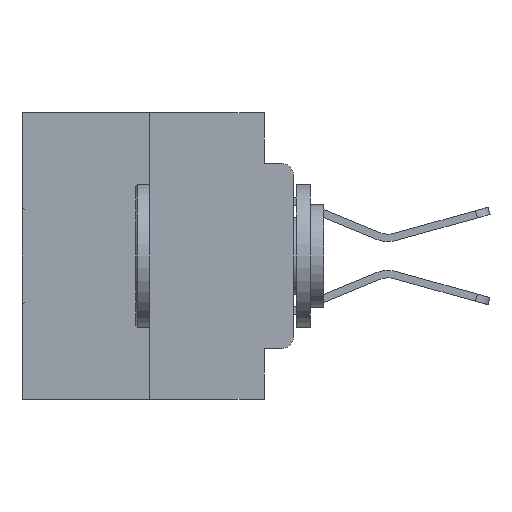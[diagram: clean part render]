
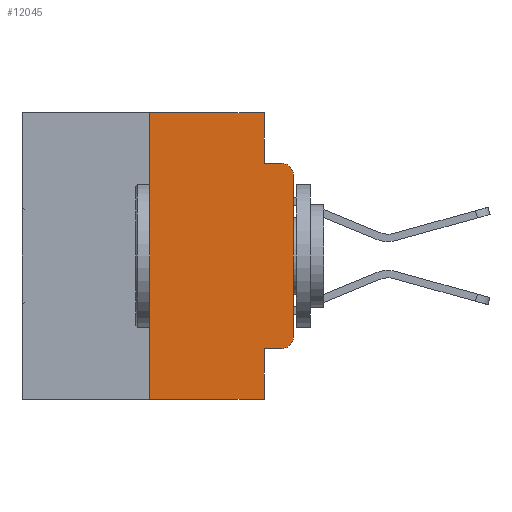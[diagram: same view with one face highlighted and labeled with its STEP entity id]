
A CAD part, left-side view. The second image highlights one B-rep face of the part: STEP entity #12045.
In plain terms, the highlighted planar face has unit normal (-1, 0, 0).
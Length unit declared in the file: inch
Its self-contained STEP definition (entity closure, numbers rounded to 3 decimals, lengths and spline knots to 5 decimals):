
#248 = ORIENTED_EDGE ( 'NONE', *, *, #29939, .F. ) ;
#392 = CARTESIAN_POINT ( 'NONE',  ( 0., 0.25, 0. ) ) ;
#1070 = VERTEX_POINT ( 'NONE', #29935 ) ;
#1841 = VECTOR ( 'NONE', #20340, 39.37008 ) ;
#1913 = CARTESIAN_POINT ( 'NONE',  ( 0., 0.051, -0.0885 ) ) ;
#2351 = CIRCLE ( 'NONE', #13292, 0.02 ) ;
#2921 = CARTESIAN_POINT ( 'NONE',  ( 0., 0.051, -0.4115 ) ) ;
#3362 = CIRCLE ( 'NONE', #20977, 0.02 ) ;
#3447 = ORIENTED_EDGE ( 'NONE', *, *, #20067, .F. ) ;
#3627 = CARTESIAN_POINT ( 'NONE',  ( 0., 0., -0.1085 ) ) ;
#3645 = VECTOR ( 'NONE', #14641, 39.37008 ) ;
#3833 = ORIENTED_EDGE ( 'NONE', *, *, #9875, .T. ) ;
#3964 = CARTESIAN_POINT ( 'NONE',  ( 0., 0.25, 0. ) ) ;
#4243 = ORIENTED_EDGE ( 'NONE', *, *, #16883, .T. ) ;
#4433 = LINE ( 'NONE', #17026, #3645 ) ;
#4945 = DIRECTION ( 'NONE',  ( 0., 0., -1. ) ) ;
#5518 = LINE ( 'NONE', #28507, #30923 ) ;
#5643 = CARTESIAN_POINT ( 'NONE',  ( 0., 0.051, -0.5 ) ) ;
#6597 = VECTOR ( 'NONE', #8872, 39.37008 ) ;
#6677 = VERTEX_POINT ( 'NONE', #2921 ) ;
#7301 = EDGE_CURVE ( 'NONE', #14435, #19936, #5518, .T. ) ;
#7581 = CARTESIAN_POINT ( 'NONE',  ( 0., 0.051, 0. ) ) ;
#8117 = VERTEX_POINT ( 'NONE', #5643 ) ;
#8255 = EDGE_CURVE ( 'NONE', #21216, #1070, #2351, .T. ) ;
#8353 = LINE ( 'NONE', #15565, #1841 ) ;
#8384 = ORIENTED_EDGE ( 'NONE', *, *, #28106, .F. ) ;
#8458 = CARTESIAN_POINT ( 'NONE',  ( 0., 0.051, 0. ) ) ;
#8872 = DIRECTION ( 'NONE',  ( 0., 0., -1. ) ) ;
#9291 = CARTESIAN_POINT ( 'NONE',  ( 0., 0.02, -0.4115 ) ) ;
#9875 = EDGE_CURVE ( 'NONE', #13082, #21216, #8353, .T. ) ;
#10429 = LINE ( 'NONE', #13683, #28762 ) ;
#11881 = DIRECTION ( 'NONE',  ( -1., 0., 0. ) ) ;
#11978 = CARTESIAN_POINT ( 'NONE',  ( 0., 0.473, 0. ) ) ;
#12045 = ADVANCED_FACE ( 'NONE', ( #12882 ), #16904, .F. ) ;
#12492 = DIRECTION ( 'NONE',  ( 0., -1., 0. ) ) ;
#12882 = FACE_OUTER_BOUND ( 'NONE', #13232, .T. ) ;
#13082 = VERTEX_POINT ( 'NONE', #24380 ) ;
#13232 = EDGE_LOOP ( 'NONE', ( #3833, #17347, #248, #13244, #26715, #8384, #21095, #3447, #22597, #4243 ) ) ;
#13244 = ORIENTED_EDGE ( 'NONE', *, *, #29693, .F. ) ;
#13292 = AXIS2_PLACEMENT_3D ( 'NONE', #27724, #13378, #30105 ) ;
#13378 = DIRECTION ( 'NONE',  ( -1., 0., 0. ) ) ;
#13556 = DIRECTION ( 'NONE',  ( 0., 0., 1. ) ) ;
#13683 = CARTESIAN_POINT ( 'NONE',  ( 0., 0.473, -0.5 ) ) ;
#14181 = DIRECTION ( 'NONE',  ( 0., -1., 0. ) ) ;
#14435 = VERTEX_POINT ( 'NONE', #392 ) ;
#14641 = DIRECTION ( 'NONE',  ( 0., -1., 0. ) ) ;
#15565 = CARTESIAN_POINT ( 'NONE',  ( 0., 0., 0. ) ) ;
#16262 = VERTEX_POINT ( 'NONE', #9291 ) ;
#16663 = VERTEX_POINT ( 'NONE', #20560 ) ;
#16883 = EDGE_CURVE ( 'NONE', #16262, #13082, #3362, .T. ) ;
#16904 = PLANE ( 'NONE',  #25812 ) ;
#17026 = CARTESIAN_POINT ( 'NONE',  ( 0., 0.051, -0.4115 ) ) ;
#17347 = ORIENTED_EDGE ( 'NONE', *, *, #8255, .T. ) ;
#18470 = EDGE_CURVE ( 'NONE', #6677, #16262, #4433, .T. ) ;
#19302 = DIRECTION ( 'NONE',  ( 1., 0., 0. ) ) ;
#19936 = VERTEX_POINT ( 'NONE', #8458 ) ;
#20067 = EDGE_CURVE ( 'NONE', #6677, #8117, #26420, .T. ) ;
#20340 = DIRECTION ( 'NONE',  ( 0., 0., 1. ) ) ;
#20560 = CARTESIAN_POINT ( 'NONE',  ( 0., 0.25, -0.5 ) ) ;
#20977 = AXIS2_PLACEMENT_3D ( 'NONE', #26201, #11881, #28626 ) ;
#21095 = ORIENTED_EDGE ( 'NONE', *, *, #25708, .T. ) ;
#21216 = VERTEX_POINT ( 'NONE', #3627 ) ;
#21858 = LINE ( 'NONE', #7581, #27489 ) ;
#22597 = ORIENTED_EDGE ( 'NONE', *, *, #18470, .T. ) ;
#24380 = CARTESIAN_POINT ( 'NONE',  ( 0., 0., -0.3915 ) ) ;
#24541 = LINE ( 'NONE', #3964, #30844 ) ;
#25602 = CARTESIAN_POINT ( 'NONE',  ( 0., 0.051, 0. ) ) ;
#25708 = EDGE_CURVE ( 'NONE', #16663, #8117, #10429, .T. ) ;
#25812 = AXIS2_PLACEMENT_3D ( 'NONE', #11978, #19302, #4945 ) ;
#26201 = CARTESIAN_POINT ( 'NONE',  ( 0., 0.02, -0.3915 ) ) ;
#26246 = VECTOR ( 'NONE', #12492, 39.37008 ) ;
#26420 = LINE ( 'NONE', #25602, #6597 ) ;
#26715 = ORIENTED_EDGE ( 'NONE', *, *, #7301, .F. ) ;
#26999 = LINE ( 'NONE', #29329, #26246 ) ;
#27489 = VECTOR ( 'NONE', #29133, 39.37008 ) ;
#27544 = VERTEX_POINT ( 'NONE', #1913 ) ;
#27724 = CARTESIAN_POINT ( 'NONE',  ( 0., 0.02, -0.1085 ) ) ;
#27998 = DIRECTION ( 'NONE',  ( 0., -1., 0. ) ) ;
#28106 = EDGE_CURVE ( 'NONE', #16663, #14435, #24541, .T. ) ;
#28507 = CARTESIAN_POINT ( 'NONE',  ( 0., 0.473, 0. ) ) ;
#28626 = DIRECTION ( 'NONE',  ( 0., 0., -1. ) ) ;
#28762 = VECTOR ( 'NONE', #27998, 39.37008 ) ;
#29133 = DIRECTION ( 'NONE',  ( 0., 0., -1. ) ) ;
#29329 = CARTESIAN_POINT ( 'NONE',  ( 0., 0.051, -0.0885 ) ) ;
#29693 = EDGE_CURVE ( 'NONE', #19936, #27544, #21858, .T. ) ;
#29935 = CARTESIAN_POINT ( 'NONE',  ( 0., 0.02, -0.0885 ) ) ;
#29939 = EDGE_CURVE ( 'NONE', #27544, #1070, #26999, .T. ) ;
#30105 = DIRECTION ( 'NONE',  ( 0., 0., -1. ) ) ;
#30844 = VECTOR ( 'NONE', #13556, 39.37008 ) ;
#30923 = VECTOR ( 'NONE', #14181, 39.37008 ) ;
